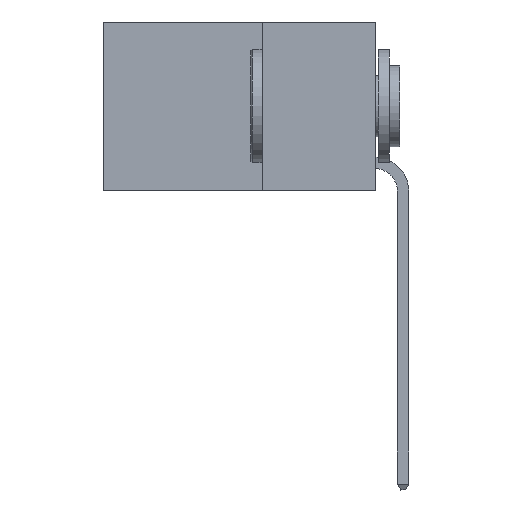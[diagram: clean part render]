
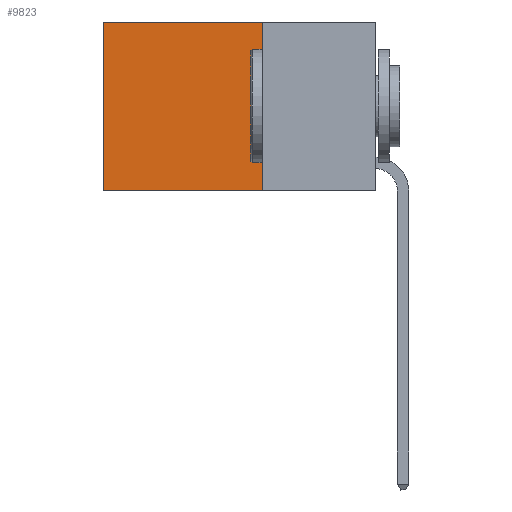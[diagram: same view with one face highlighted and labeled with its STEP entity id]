
A CAD part, left-side view. The second image highlights one B-rep face of the part: STEP entity #9823.
In plain terms, the highlighted planar face has unit normal (-1, 0, 0).
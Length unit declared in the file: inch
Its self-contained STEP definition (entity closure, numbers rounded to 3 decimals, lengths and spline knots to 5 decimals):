
#234 = FACE_OUTER_BOUND ( 'NONE', #5798, .T. ) ;
#672 = CARTESIAN_POINT ( 'NONE',  ( 0.2625, 0.6, 0. ) ) ;
#1577 = PLANE ( 'NONE',  #12796 ) ;
#1767 = DIRECTION ( 'NONE',  ( 0., 0., -1. ) ) ;
#1904 = CARTESIAN_POINT ( 'NONE',  ( 0.2625, 0.25, 0. ) ) ;
#2742 = CARTESIAN_POINT ( 'NONE',  ( 0.2625, 0.25, -0.37 ) ) ;
#2928 = LINE ( 'NONE', #2742, #11785 ) ;
#3776 = CARTESIAN_POINT ( 'NONE',  ( 0.2625, 0.25, 0. ) ) ;
#4537 = EDGE_CURVE ( 'NONE', #13074, #8927, #7535, .T. ) ;
#4595 = VECTOR ( 'NONE', #1767, 39.37008 ) ;
#5000 = ORIENTED_EDGE ( 'NONE', *, *, #4537, .T. ) ;
#5151 = ORIENTED_EDGE ( 'NONE', *, *, #10914, .F. ) ;
#5162 = ORIENTED_EDGE ( 'NONE', *, *, #5723, .F. ) ;
#5179 = ORIENTED_EDGE ( 'NONE', *, *, #12917, .T. ) ;
#5429 = VECTOR ( 'NONE', #11285, 39.37008 ) ;
#5514 = VERTEX_POINT ( 'NONE', #6540 ) ;
#5723 = EDGE_CURVE ( 'NONE', #8203, #5514, #13073, .T. ) ;
#5798 = EDGE_LOOP ( 'NONE', ( #5000, #5151, #5162, #5179 ) ) ;
#6016 = CARTESIAN_POINT ( 'NONE',  ( 0.2625, 0.25, 0. ) ) ;
#6156 = VECTOR ( 'NONE', #8520, 39.37008 ) ;
#6371 = CARTESIAN_POINT ( 'NONE',  ( 0.2625, 0.25, 0. ) ) ;
#6540 = CARTESIAN_POINT ( 'NONE',  ( 0.2625, 0.25, -0.37 ) ) ;
#7129 = DIRECTION ( 'NONE',  ( 0., 0., -1. ) ) ;
#7535 = LINE ( 'NONE', #672, #4595 ) ;
#8203 = VERTEX_POINT ( 'NONE', #6371 ) ;
#8520 = DIRECTION ( 'NONE',  ( 0., 1., 0. ) ) ;
#8927 = VERTEX_POINT ( 'NONE', #13675 ) ;
#9823 = ADVANCED_FACE ( 'NONE', ( #234 ), #1577, .F. ) ;
#10914 = EDGE_CURVE ( 'NONE', #5514, #8927, #2928, .T. ) ;
#11285 = DIRECTION ( 'NONE',  ( 0., 0., -1. ) ) ;
#11714 = LINE ( 'NONE', #1904, #6156 ) ;
#11785 = VECTOR ( 'NONE', #13230, 39.37008 ) ;
#12246 = CARTESIAN_POINT ( 'NONE',  ( 0.2625, 0.6, 0. ) ) ;
#12796 = AXIS2_PLACEMENT_3D ( 'NONE', #6016, #13218, #7129 ) ;
#12917 = EDGE_CURVE ( 'NONE', #8203, #13074, #11714, .T. ) ;
#13073 = LINE ( 'NONE', #3776, #5429 ) ;
#13074 = VERTEX_POINT ( 'NONE', #12246 ) ;
#13218 = DIRECTION ( 'NONE',  ( 1., 0., 0. ) ) ;
#13230 = DIRECTION ( 'NONE',  ( 0., 1., 0. ) ) ;
#13675 = CARTESIAN_POINT ( 'NONE',  ( 0.2625, 0.6, -0.37 ) ) ;
